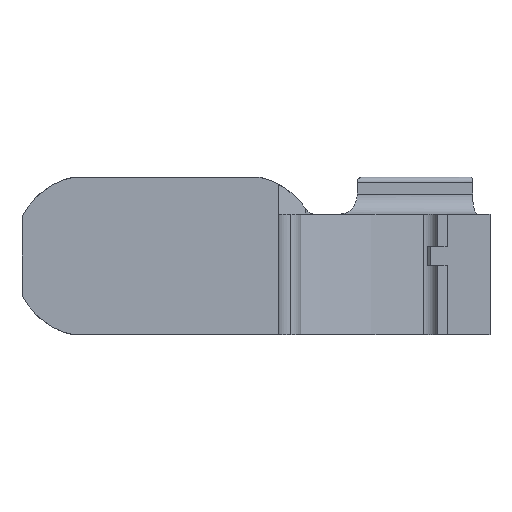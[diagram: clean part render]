
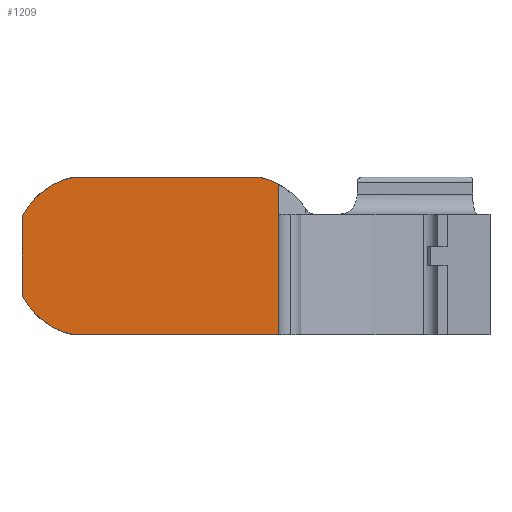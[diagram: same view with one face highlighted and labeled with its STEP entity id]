
A CAD part, front view. The second image highlights one B-rep face of the part: STEP entity #1209.
In plain terms, the highlighted planar face has unit normal (0, -1, 0).
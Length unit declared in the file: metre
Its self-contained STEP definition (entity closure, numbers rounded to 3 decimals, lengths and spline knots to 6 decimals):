
#103=CIRCLE('',#1343,0.005934);
#104=CIRCLE('',#1344,0.005934);
#105=CIRCLE('',#1345,0.005934);
#152=FACE_OUTER_BOUND('',#215,.T.);
#215=EDGE_LOOP('',(#1032,#1033,#1034,#1035,#1036,#1037,#1038));
#253=LINE('',#1796,#372);
#271=LINE('',#1856,#390);
#334=LINE('',#2038,#453);
#335=LINE('',#2041,#454);
#372=VECTOR('',#1429,0.014606);
#390=VECTOR('',#1481,0.016179);
#453=VECTOR('',#1656,0.006173);
#454=VECTOR('',#1659,0.011874);
#503=VERTEX_POINT('',#1793);
#504=VERTEX_POINT('',#1795);
#528=VERTEX_POINT('',#1853);
#529=VERTEX_POINT('',#1855);
#577=VERTEX_POINT('',#2035);
#578=VERTEX_POINT('',#2037);
#579=VERTEX_POINT('',#2040);
#625=EDGE_CURVE('',#503,#504,#253,.T.);
#655=EDGE_CURVE('',#529,#528,#271,.T.);
#740=EDGE_CURVE('',#503,#577,#103,.F.);
#741=EDGE_CURVE('',#577,#578,#334,.T.);
#742=EDGE_CURVE('',#578,#529,#104,.F.);
#743=EDGE_CURVE('',#579,#528,#335,.T.);
#744=EDGE_CURVE('',#504,#579,#105,.T.);
#1032=ORIENTED_EDGE('',*,*,#625,.F.);
#1033=ORIENTED_EDGE('',*,*,#740,.T.);
#1034=ORIENTED_EDGE('',*,*,#741,.T.);
#1035=ORIENTED_EDGE('',*,*,#742,.T.);
#1036=ORIENTED_EDGE('',*,*,#655,.T.);
#1037=ORIENTED_EDGE('',*,*,#743,.F.);
#1038=ORIENTED_EDGE('',*,*,#744,.F.);
#1157=PLANE('',#1342);
#1209=ADVANCED_FACE('',(#152),#1157,.F.);
#1342=AXIS2_PLACEMENT_3D('',#2034,#1652,#1653);
#1343=AXIS2_PLACEMENT_3D('',#2036,#1654,#1655);
#1344=AXIS2_PLACEMENT_3D('',#2039,#1657,#1658);
#1345=AXIS2_PLACEMENT_3D('',#2042,#1660,#1661);
#1429=DIRECTION('',(1.,0.,0.));
#1481=DIRECTION('',(1.,0.,0.));
#1652=DIRECTION('center_axis',(0.,1.,0.));
#1653=DIRECTION('ref_axis',(-1.,0.,0.));
#1654=DIRECTION('center_axis',(0.,1.,0.));
#1655=DIRECTION('ref_axis',(-1.,0.,0.));
#1656=DIRECTION('',(0.,0.,-1.));
#1657=DIRECTION('center_axis',(0.,1.,0.));
#1658=DIRECTION('ref_axis',(-1.,0.,0.));
#1659=DIRECTION('',(0.,0.,-1.));
#1660=DIRECTION('center_axis',(0.,1.,0.));
#1661=DIRECTION('ref_axis',(-1.,0.,0.));
#1793=CARTESIAN_POINT('',(-0.00605,-0.009525,0.00562));
#1795=CARTESIAN_POINT('',(0.008555,-0.009525,0.00562));
#1796=CARTESIAN_POINT('',(-0.00605,-0.009525,0.00562));
#1853=CARTESIAN_POINT('',(0.010128,-0.009525,-0.006826));
#1855=CARTESIAN_POINT('',(-0.00605,-0.009525,-0.006826));
#1856=CARTESIAN_POINT('',(-0.00605,-0.009525,-0.006826));
#2034=CARTESIAN_POINT('Origin',(-0.000603,-0.009525,0.00562));
#2035=CARTESIAN_POINT('',(-0.010128,-0.009525,0.002483));
#2036=CARTESIAN_POINT('Origin',(-0.004829,-0.009525,-0.000187));
#2037=CARTESIAN_POINT('',(-0.010128,-0.009525,-0.00369));
#2038=CARTESIAN_POINT('',(-0.010128,-0.009525,0.002483));
#2039=CARTESIAN_POINT('Origin',(-0.004829,-0.009525,-0.001019));
#2040=CARTESIAN_POINT('',(0.010128,-0.009525,0.005048));
#2041=CARTESIAN_POINT('',(0.010128,-0.009525,0.005048));
#2042=CARTESIAN_POINT('Origin',(0.007334,-0.009525,-0.000187));
